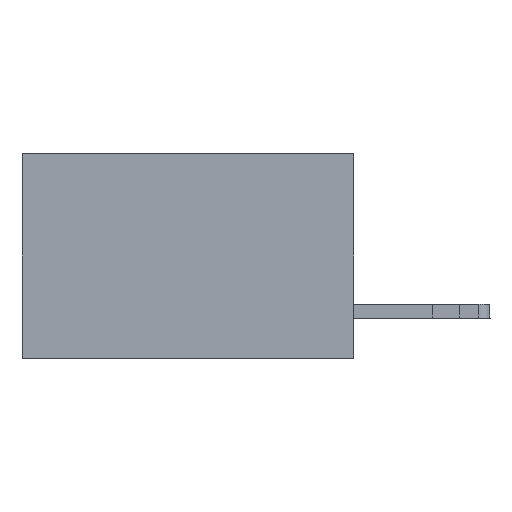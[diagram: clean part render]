
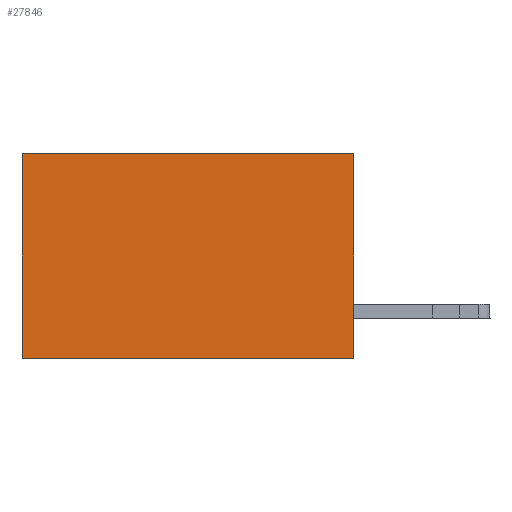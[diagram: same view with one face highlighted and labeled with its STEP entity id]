
A CAD part, left-side view. The second image highlights one B-rep face of the part: STEP entity #27846.
In plain terms, the highlighted planar face has unit normal (-1, 0, 0).
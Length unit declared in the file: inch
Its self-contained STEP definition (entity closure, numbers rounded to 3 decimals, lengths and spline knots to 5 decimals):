
#3785 = EDGE_CURVE ( 'NONE', #24602, #24724, #7551, .T. ) ;
#5219 = EDGE_CURVE ( 'NONE', #24602, #22323, #8288, .T. ) ;
#5398 = CARTESIAN_POINT ( 'NONE',  ( 0.2875, 0.6, 0. ) ) ;
#5861 = DIRECTION ( 'NONE',  ( 1., 0., 0. ) ) ;
#5948 = VERTEX_POINT ( 'NONE', #6428 ) ;
#6428 = CARTESIAN_POINT ( 'NONE',  ( 0.2875, 0.6, -0.37 ) ) ;
#6971 = ORIENTED_EDGE ( 'NONE', *, *, #10051, .T. ) ;
#7426 = EDGE_CURVE ( 'NONE', #22323, #5948, #27832, .T. ) ;
#7551 = LINE ( 'NONE', #28782, #12464 ) ;
#8288 = LINE ( 'NONE', #24406, #27558 ) ;
#8327 = FACE_OUTER_BOUND ( 'NONE', #8403, .T. ) ;
#8351 = VECTOR ( 'NONE', #22464, 39.37008 ) ;
#8403 = EDGE_LOOP ( 'NONE', ( #6971, #23246, #10789, #30767 ) ) ;
#10051 = EDGE_CURVE ( 'NONE', #24724, #5948, #18130, .T. ) ;
#10789 = ORIENTED_EDGE ( 'NONE', *, *, #5219, .F. ) ;
#12464 = VECTOR ( 'NONE', #14366, 39.37008 ) ;
#13440 = CARTESIAN_POINT ( 'NONE',  ( 0.2875, 0.6, 0. ) ) ;
#14366 = DIRECTION ( 'NONE',  ( 0., 1., 0. ) ) ;
#17423 = DIRECTION ( 'NONE',  ( 0., 0., -1. ) ) ;
#18130 = LINE ( 'NONE', #5398, #8351 ) ;
#18152 = CARTESIAN_POINT ( 'NONE',  ( 0.2875, 0., 0. ) ) ;
#22323 = VERTEX_POINT ( 'NONE', #24122 ) ;
#22464 = DIRECTION ( 'NONE',  ( 0., 0., -1. ) ) ;
#22711 = DIRECTION ( 'NONE',  ( 0., 0., -1. ) ) ;
#23246 = ORIENTED_EDGE ( 'NONE', *, *, #7426, .F. ) ;
#24122 = CARTESIAN_POINT ( 'NONE',  ( 0.2875, 0., -0.37 ) ) ;
#24406 = CARTESIAN_POINT ( 'NONE',  ( 0.2875, 0., 0. ) ) ;
#24602 = VERTEX_POINT ( 'NONE', #30285 ) ;
#24724 = VERTEX_POINT ( 'NONE', #13440 ) ;
#25013 = DIRECTION ( 'NONE',  ( 0., 1., 0. ) ) ;
#27558 = VECTOR ( 'NONE', #17423, 39.37008 ) ;
#27570 = CARTESIAN_POINT ( 'NONE',  ( 0.2875, 0., -0.37 ) ) ;
#27832 = LINE ( 'NONE', #27570, #28611 ) ;
#27846 = ADVANCED_FACE ( 'NONE', ( #8327 ), #30179, .F. ) ;
#28611 = VECTOR ( 'NONE', #25013, 39.37008 ) ;
#28782 = CARTESIAN_POINT ( 'NONE',  ( 0.2875, 0., 0. ) ) ;
#30179 = PLANE ( 'NONE',  #31163 ) ;
#30285 = CARTESIAN_POINT ( 'NONE',  ( 0.2875, 0., 0. ) ) ;
#30767 = ORIENTED_EDGE ( 'NONE', *, *, #3785, .T. ) ;
#31163 = AXIS2_PLACEMENT_3D ( 'NONE', #18152, #5861, #22711 ) ;
